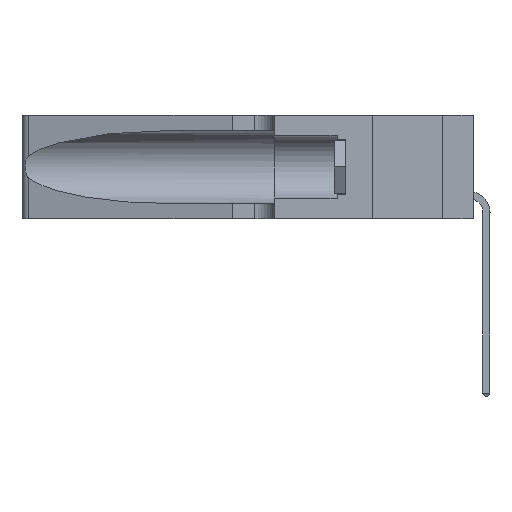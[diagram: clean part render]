
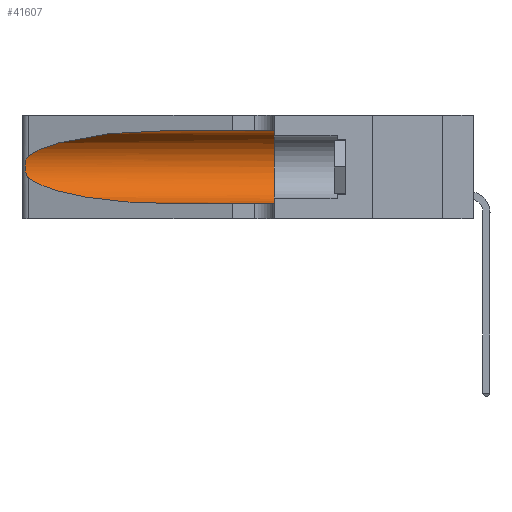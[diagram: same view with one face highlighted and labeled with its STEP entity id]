
A CAD part, left-side view. The second image highlights one B-rep face of the part: STEP entity #41607.
In plain terms, the highlighted cylindrical face has radius 3.308 mm (diameter 6.617 mm), a partial arc.
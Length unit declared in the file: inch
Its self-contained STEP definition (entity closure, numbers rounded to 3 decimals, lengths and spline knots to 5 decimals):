
#456 = VERTEX_POINT ( 'NONE', #26014 ) ;
#3171 = DIRECTION ( 'NONE',  ( 0., -1., 0. ) ) ;
#4191 = CARTESIAN_POINT ( 'NONE',  ( 0.26018, 1.23835, 0.19895 ) ) ;
#4344 = CARTESIAN_POINT ( 'NONE',  ( 0.26017, 1.23833, 0.17102 ) ) ;
#4486 = DIRECTION ( 'NONE',  ( 0., 0., -1. ) ) ;
#4496 = CYLINDRICAL_SURFACE ( 'NONE', #36579, 0.13025 ) ;
#4631 = CARTESIAN_POINT ( 'NONE',  ( 0.25555, 1.22994, 0.2215 ) ) ;
#4795 = CARTESIAN_POINT ( 'NONE',  ( 0.26075, 1.23896, 0.178 ) ) ;
#5609 = FACE_OUTER_BOUND ( 'NONE', #42420, .T. ) ;
#5738 = LINE ( 'NONE', #24505, #41623 ) ;
#5817 = EDGE_CURVE ( 'NONE', #14366, #46168, #29651, .T. ) ;
#8233 = CARTESIAN_POINT ( 'NONE',  ( 0.25639, 1.23186, 0.15144 ) ) ;
#8383 = CARTESIAN_POINT ( 'NONE',  ( 0.25555, 1.22993, 0.14849 ) ) ;
#9267 = ORIENTED_EDGE ( 'NONE', *, *, #41083, .T. ) ;
#9548 = DIRECTION ( 'NONE',  ( 0., -1., 0. ) ) ;
#9744 = CARTESIAN_POINT ( 'NONE',  ( 0.2373, 1.15595, 0.28018 ) ) ;
#11585 = B_SPLINE_CURVE_WITH_KNOTS ( 'NONE', 3,
 ( #22423, #4631, #40019, #18999, #40336, #4191, #29643, #4795, #4344, #18522, #21958, #8233, #8383, #43624 ),
 .UNSPECIFIED., .F., .F.,
 ( 4, 2, 2, 2, 2, 2, 4 ),
 ( 0., 0.00027, 0.00053, 0.00107, 0.0016, 0.00187, 0.00214 ),
 .UNSPECIFIED. ) ;
#13843 = CIRCLE ( 'NONE', #38693, 0.13025 ) ;
#14366 = VERTEX_POINT ( 'NONE', #23369 ) ;
#16172 = VERTEX_POINT ( 'NONE', #25779 ) ;
#17957 = VERTEX_POINT ( 'NONE', #38416 ) ;
#18522 = CARTESIAN_POINT ( 'NONE',  ( 0.25856, 1.23593, 0.16098 ) ) ;
#18999 = CARTESIAN_POINT ( 'NONE',  ( 0.25787, 1.23484, 0.2124 ) ) ;
#20803 = ORIENTED_EDGE ( 'NONE', *, *, #45128, .T. ) ;
#21958 = CARTESIAN_POINT ( 'NONE',  ( 0.25789, 1.23486, 0.15765 ) ) ;
#22055 = CARTESIAN_POINT ( 'NONE',  ( 0.25487, 1.22718, 0.14631 ) ) ;
#22257 = ORIENTED_EDGE ( 'NONE', *, *, #45642, .T. ) ;
#22423 = CARTESIAN_POINT ( 'NONE',  ( 0.25487, 1.22718, 0.22369 ) ) ;
#22971 = VECTOR ( 'NONE', #9548, 39.37008 ) ;
#23369 = CARTESIAN_POINT ( 'NONE',  ( 0.1305, 0.72297, 0.31525 ) ) ;
#23744 = CARTESIAN_POINT ( 'NONE',  ( 0.18966, 0.96281, 0.31525 ) ) ;
#23991 = ORIENTED_EDGE ( 'NONE', *, *, #31957, .F. ) ;
#24505 = CARTESIAN_POINT ( 'NONE',  ( 0.1305, 1.61858, 0.31525 ) ) ;
#25779 = CARTESIAN_POINT ( 'NONE',  ( 0.25487, 1.22718, 0.14631 ) ) ;
#26014 = CARTESIAN_POINT ( 'NONE',  ( 0.1305, 0.72297, 0.05475 ) ) ;
#26152 = CARTESIAN_POINT ( 'NONE',  ( 0.1305, 1.61858, 0.185 ) ) ;
#28959 = EDGE_CURVE ( 'NONE', #14366, #37146, #5738, .T. ) ;
#29643 = CARTESIAN_POINT ( 'NONE',  ( 0.26075, 1.23896, 0.19203 ) ) ;
#29651 =( BOUNDED_CURVE ( )  B_SPLINE_CURVE ( 3, ( #38218, #23744, #9744, #34149 ),
 .UNSPECIFIED., .F., .T. ) 
 B_SPLINE_CURVE_WITH_KNOTS ( ( 4, 4 ),
 ( 1.5708, 2.84003 ),
 .UNSPECIFIED. ) 
 CURVE ( )  GEOMETRIC_REPRESENTATION_ITEM ( )  RATIONAL_B_SPLINE_CURVE ( ( 1., 0.87, 0.87, 1. ) ) 
 REPRESENTATION_ITEM ( '' )  );
#30127 = DIRECTION ( 'NONE',  ( 0., 1., 0. ) ) ;
#31707 =( BOUNDED_CURVE ( )  B_SPLINE_CURVE ( 3, ( #22055, #32279, #36351, #39955 ),
 .UNSPECIFIED., .F., .F. ) 
 B_SPLINE_CURVE_WITH_KNOTS ( ( 4, 4 ),
 ( 3.44316, 4.71239 ),
 .UNSPECIFIED. ) 
 CURVE ( )  GEOMETRIC_REPRESENTATION_ITEM ( )  RATIONAL_B_SPLINE_CURVE ( ( 1., 0.87, 0.87, 1. ) ) 
 REPRESENTATION_ITEM ( '' )  );
#31957 = EDGE_CURVE ( 'NONE', #37146, #17957, #13843, .T. ) ;
#32279 = CARTESIAN_POINT ( 'NONE',  ( 0.2373, 1.15595, 0.08982 ) ) ;
#34149 = CARTESIAN_POINT ( 'NONE',  ( 0.25487, 1.22718, 0.22369 ) ) ;
#34405 = CARTESIAN_POINT ( 'NONE',  ( 0.1305, 0.35, 0.31525 ) ) ;
#36351 = CARTESIAN_POINT ( 'NONE',  ( 0.18966, 0.96281, 0.05475 ) ) ;
#36579 = AXIS2_PLACEMENT_3D ( 'NONE', #26152, #36714, #4486 ) ;
#36714 = DIRECTION ( 'NONE',  ( 0., -1., 0. ) ) ;
#37146 = VERTEX_POINT ( 'NONE', #34405 ) ;
#37275 = CARTESIAN_POINT ( 'NONE',  ( 0.25487, 1.22718, 0.22369 ) ) ;
#38218 = CARTESIAN_POINT ( 'NONE',  ( 0.1305, 0.72297, 0.31525 ) ) ;
#38416 = CARTESIAN_POINT ( 'NONE',  ( 0.1305, 0.35, 0.05475 ) ) ;
#38419 = DIRECTION ( 'NONE',  ( 0., 0., 1. ) ) ;
#38693 = AXIS2_PLACEMENT_3D ( 'NONE', #40351, #30127, #38419 ) ;
#39955 = CARTESIAN_POINT ( 'NONE',  ( 0.1305, 0.72297, 0.05475 ) ) ;
#40019 = CARTESIAN_POINT ( 'NONE',  ( 0.25639, 1.23184, 0.21858 ) ) ;
#40336 = CARTESIAN_POINT ( 'NONE',  ( 0.25854, 1.2359, 0.20912 ) ) ;
#40351 = CARTESIAN_POINT ( 'NONE',  ( 0.1305, 0.35, 0.185 ) ) ;
#41083 = EDGE_CURVE ( 'NONE', #456, #17957, #42128, .T. ) ;
#41607 = ADVANCED_FACE ( 'NONE', ( #5609 ), #4496, .F. ) ;
#41623 = VECTOR ( 'NONE', #3171, 39.37008 ) ;
#42128 = LINE ( 'NONE', #45412, #22971 ) ;
#42420 = EDGE_LOOP ( 'NONE', ( #42787, #20803, #22257, #9267, #23991, #42556 ) ) ;
#42556 = ORIENTED_EDGE ( 'NONE', *, *, #28959, .F. ) ;
#42787 = ORIENTED_EDGE ( 'NONE', *, *, #5817, .T. ) ;
#43624 = CARTESIAN_POINT ( 'NONE',  ( 0.25487, 1.22718, 0.14631 ) ) ;
#45128 = EDGE_CURVE ( 'NONE', #46168, #16172, #11585, .T. ) ;
#45412 = CARTESIAN_POINT ( 'NONE',  ( 0.1305, 1.61858, 0.05475 ) ) ;
#45642 = EDGE_CURVE ( 'NONE', #16172, #456, #31707, .T. ) ;
#46168 = VERTEX_POINT ( 'NONE', #37275 ) ;
